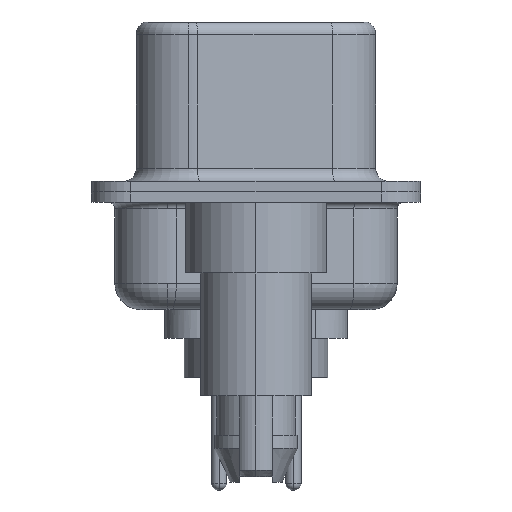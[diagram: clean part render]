
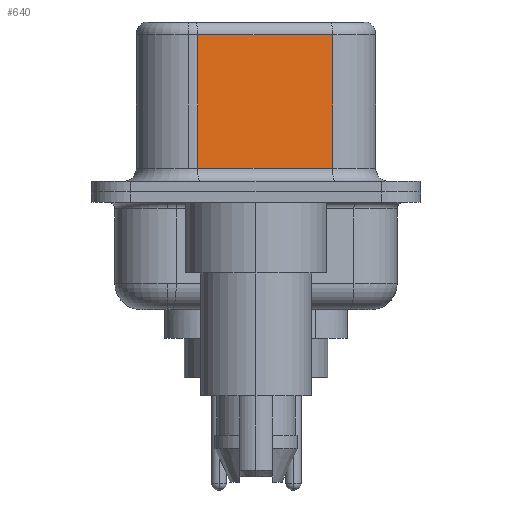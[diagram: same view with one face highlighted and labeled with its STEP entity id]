
A CAD part, left-side view. The second image highlights one B-rep face of the part: STEP entity #640.
In plain terms, the highlighted planar face has unit normal (-0.985, -0.174, 0).
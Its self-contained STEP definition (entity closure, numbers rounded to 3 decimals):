
#24 = DIRECTION ( 'NONE',  ( 0.174, -0.985, 0. ) ) ;
#248 = CARTESIAN_POINT ( 'NONE',  ( 4.565, -2.927, 0.9 ) ) ;
#625 = LINE ( 'NONE', #248, #3683 ) ;
#640 = ADVANCED_FACE ( 'NONE', ( #2131 ), #13462, .F. ) ;
#839 = EDGE_LOOP ( 'NONE', ( #7397, #2174, #7577, #10839 ) ) ;
#1137 = LINE ( 'NONE', #2444, #14298 ) ;
#1241 = LINE ( 'NONE', #15132, #8824 ) ;
#2131 = FACE_OUTER_BOUND ( 'NONE', #839, .T. ) ;
#2174 = ORIENTED_EDGE ( 'NONE', *, *, #10301, .T. ) ;
#2444 = CARTESIAN_POINT ( 'NONE',  ( 3.655, 2.233, 6.52 ) ) ;
#3116 = DIRECTION ( 'NONE',  ( 0.985, 0.174, 0. ) ) ;
#3125 = CARTESIAN_POINT ( 'NONE',  ( 4.565, -2.927, 6.02 ) ) ;
#3683 = VECTOR ( 'NONE', #24, 1000. ) ;
#4127 = CARTESIAN_POINT ( 'NONE',  ( 4.565, -2.927, 6.52 ) ) ;
#4739 = CARTESIAN_POINT ( 'NONE',  ( 4.565, -2.927, 6.02 ) ) ;
#4953 = VERTEX_POINT ( 'NONE', #13320 ) ;
#5564 = CARTESIAN_POINT ( 'NONE',  ( 4.565, -2.927, 0.9 ) ) ;
#5951 = DIRECTION ( 'NONE',  ( -0.174, 0.985, 0. ) ) ;
#7397 = ORIENTED_EDGE ( 'NONE', *, *, #8809, .F. ) ;
#7577 = ORIENTED_EDGE ( 'NONE', *, *, #9879, .T. ) ;
#8565 = EDGE_CURVE ( 'NONE', #4953, #11336, #625, .T. ) ;
#8809 = EDGE_CURVE ( 'NONE', #9585, #11336, #1241, .T. ) ;
#8824 = VECTOR ( 'NONE', #14992, 1000. ) ;
#9130 = VECTOR ( 'NONE', #13622, 1000. ) ;
#9585 = VERTEX_POINT ( 'NONE', #3125 ) ;
#9879 = EDGE_CURVE ( 'NONE', #14957, #4953, #1137, .T. ) ;
#10301 = EDGE_CURVE ( 'NONE', #9585, #14957, #12472, .T. ) ;
#10839 = ORIENTED_EDGE ( 'NONE', *, *, #8565, .T. ) ;
#11296 = DIRECTION ( 'NONE',  ( 0., 0., -1. ) ) ;
#11336 = VERTEX_POINT ( 'NONE', #5564 ) ;
#11979 = AXIS2_PLACEMENT_3D ( 'NONE', #4127, #3116, #5951 ) ;
#12472 = LINE ( 'NONE', #4739, #9130 ) ;
#13320 = CARTESIAN_POINT ( 'NONE',  ( 3.655, 2.233, 0.9 ) ) ;
#13462 = PLANE ( 'NONE',  #11979 ) ;
#13622 = DIRECTION ( 'NONE',  ( -0.174, 0.985, 0. ) ) ;
#14298 = VECTOR ( 'NONE', #11296, 1000. ) ;
#14957 = VERTEX_POINT ( 'NONE', #15759 ) ;
#14992 = DIRECTION ( 'NONE',  ( 0., 0., -1. ) ) ;
#15132 = CARTESIAN_POINT ( 'NONE',  ( 4.565, -2.927, 6.52 ) ) ;
#15759 = CARTESIAN_POINT ( 'NONE',  ( 3.655, 2.233, 6.02 ) ) ;
